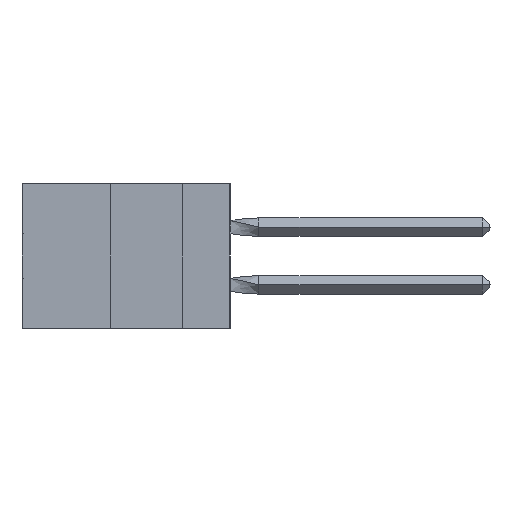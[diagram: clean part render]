
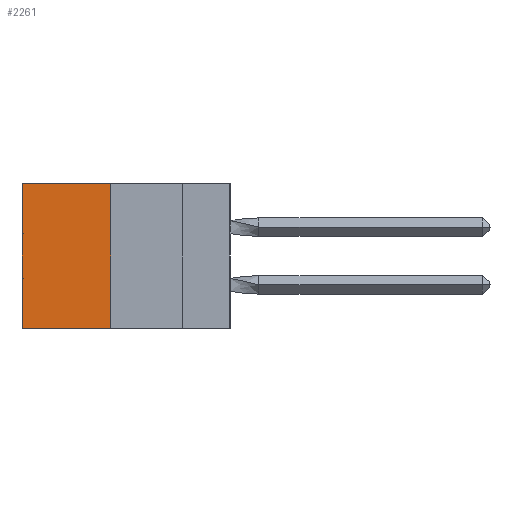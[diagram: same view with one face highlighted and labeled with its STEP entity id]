
A CAD part, left-side view. The second image highlights one B-rep face of the part: STEP entity #2261.
In plain terms, the highlighted planar face has unit normal (-1, 0, 0).
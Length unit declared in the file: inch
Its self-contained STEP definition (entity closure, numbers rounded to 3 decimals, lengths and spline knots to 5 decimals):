
#1654 = VERTEX_POINT ( 'NONE', #8047 ) ;
#1785 = CARTESIAN_POINT ( 'NONE',  ( 0.305, 0.413, -0.5 ) ) ;
#2261 = ADVANCED_FACE ( 'NONE', ( #23594 ), #28889, .F. ) ;
#3936 = ORIENTED_EDGE ( 'NONE', *, *, #21764, .T. ) ;
#7007 = ORIENTED_EDGE ( 'NONE', *, *, #23208, .F. ) ;
#7770 = DIRECTION ( 'NONE',  ( 0., 1., 0. ) ) ;
#8047 = CARTESIAN_POINT ( 'NONE',  ( 0.305, 0.413, 0. ) ) ;
#8156 = LINE ( 'NONE', #34658, #38756 ) ;
#9935 = VERTEX_POINT ( 'NONE', #13289 ) ;
#9994 = DIRECTION ( 'NONE',  ( 0., 0., -1. ) ) ;
#10309 = DIRECTION ( 'NONE',  ( 0., 0., -1. ) ) ;
#12100 = LINE ( 'NONE', #32493, #37442 ) ;
#12240 = VECTOR ( 'NONE', #35528, 39.37008 ) ;
#13289 = CARTESIAN_POINT ( 'NONE',  ( 0.305, 0.72, 0. ) ) ;
#13693 = CARTESIAN_POINT ( 'NONE',  ( 0.305, 0.413, -0.5 ) ) ;
#15790 = LINE ( 'NONE', #39477, #12240 ) ;
#17193 = VERTEX_POINT ( 'NONE', #18332 ) ;
#17995 = DIRECTION ( 'NONE',  ( 1., 0., 0. ) ) ;
#18332 = CARTESIAN_POINT ( 'NONE',  ( 0.305, 0.72, -0.5 ) ) ;
#20754 = VECTOR ( 'NONE', #31227, 39.37008 ) ;
#21764 = EDGE_CURVE ( 'NONE', #1654, #9935, #15790, .T. ) ;
#22166 = ORIENTED_EDGE ( 'NONE', *, *, #30033, .T. ) ;
#23208 = EDGE_CURVE ( 'NONE', #1654, #38956, #12100, .T. ) ;
#23594 = FACE_OUTER_BOUND ( 'NONE', #38401, .T. ) ;
#25247 = AXIS2_PLACEMENT_3D ( 'NONE', #13693, #17995, #10309 ) ;
#28889 = PLANE ( 'NONE',  #25247 ) ;
#30033 = EDGE_CURVE ( 'NONE', #9935, #17193, #48499, .T. ) ;
#31227 = DIRECTION ( 'NONE',  ( 0., 0., -1. ) ) ;
#32493 = CARTESIAN_POINT ( 'NONE',  ( 0.305, 0.413, -0.5 ) ) ;
#34658 = CARTESIAN_POINT ( 'NONE',  ( 0.305, 0.413, -0.5 ) ) ;
#35347 = EDGE_CURVE ( 'NONE', #38956, #17193, #8156, .T. ) ;
#35528 = DIRECTION ( 'NONE',  ( 0., 1., 0. ) ) ;
#37129 = ORIENTED_EDGE ( 'NONE', *, *, #35347, .F. ) ;
#37442 = VECTOR ( 'NONE', #9994, 39.37008 ) ;
#38401 = EDGE_LOOP ( 'NONE', ( #22166, #37129, #7007, #3936 ) ) ;
#38756 = VECTOR ( 'NONE', #7770, 39.37008 ) ;
#38956 = VERTEX_POINT ( 'NONE', #1785 ) ;
#39477 = CARTESIAN_POINT ( 'NONE',  ( 0.305, 0.413, 0. ) ) ;
#43989 = CARTESIAN_POINT ( 'NONE',  ( 0.305, 0.72, -0.5 ) ) ;
#48499 = LINE ( 'NONE', #43989, #20754 ) ;
